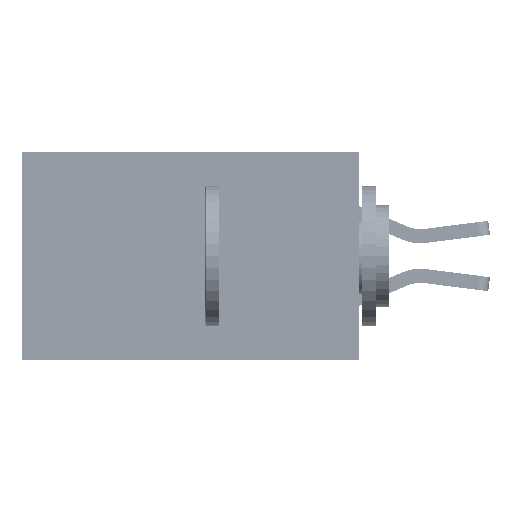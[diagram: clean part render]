
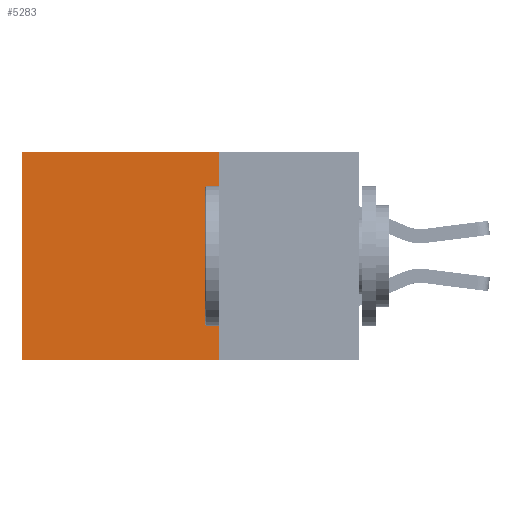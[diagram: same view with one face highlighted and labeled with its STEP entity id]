
A CAD part, left-side view. The second image highlights one B-rep face of the part: STEP entity #5283.
In plain terms, the highlighted planar face has unit normal (-1, 0, 0).
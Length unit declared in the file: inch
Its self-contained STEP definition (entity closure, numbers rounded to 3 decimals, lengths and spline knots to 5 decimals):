
#242 = VERTEX_POINT ( 'NONE', #3728 ) ;
#617 = FACE_OUTER_BOUND ( 'NONE', #26051, .T. ) ;
#1172 = EDGE_CURVE ( 'NONE', #27833, #26442, #19711, .T. ) ;
#1652 = VECTOR ( 'NONE', #17837, 39.37008 ) ;
#2261 = CARTESIAN_POINT ( 'NONE',  ( 0.2875, 0.25, -0.37 ) ) ;
#3349 = VECTOR ( 'NONE', #19250, 39.37008 ) ;
#3728 = CARTESIAN_POINT ( 'NONE',  ( 0.2875, 0.6, 0. ) ) ;
#4621 = DIRECTION ( 'NONE',  ( 0., 0., -1. ) ) ;
#5283 = ADVANCED_FACE ( 'NONE', ( #617 ), #14003, .F. ) ;
#5705 = DIRECTION ( 'NONE',  ( 1., 0., 0. ) ) ;
#5849 = EDGE_CURVE ( 'NONE', #26442, #14584, #29933, .T. ) ;
#10120 = VECTOR ( 'NONE', #17584, 39.37008 ) ;
#10176 = EDGE_CURVE ( 'NONE', #242, #14584, #37943, .T. ) ;
#12359 = DIRECTION ( 'NONE',  ( 0., 0., -1. ) ) ;
#14003 = PLANE ( 'NONE',  #40813 ) ;
#14584 = VERTEX_POINT ( 'NONE', #40375 ) ;
#17404 = ORIENTED_EDGE ( 'NONE', *, *, #31392, .T. ) ;
#17584 = DIRECTION ( 'NONE',  ( 0., 1., 0. ) ) ;
#17837 = DIRECTION ( 'NONE',  ( 0., 1., 0. ) ) ;
#18620 = LINE ( 'NONE', #33529, #10120 ) ;
#19250 = DIRECTION ( 'NONE',  ( 0., 0., -1. ) ) ;
#19290 = CARTESIAN_POINT ( 'NONE',  ( 0.2875, 0.25, -0.37 ) ) ;
#19711 = LINE ( 'NONE', #36490, #3349 ) ;
#23425 = ORIENTED_EDGE ( 'NONE', *, *, #1172, .F. ) ;
#26051 = EDGE_LOOP ( 'NONE', ( #35237, #38483, #23425, #17404 ) ) ;
#26442 = VERTEX_POINT ( 'NONE', #19290 ) ;
#26561 = CARTESIAN_POINT ( 'NONE',  ( 0.2875, 0.25, 0. ) ) ;
#27833 = VERTEX_POINT ( 'NONE', #26561 ) ;
#29933 = LINE ( 'NONE', #2261, #1652 ) ;
#31392 = EDGE_CURVE ( 'NONE', #27833, #242, #18620, .T. ) ;
#33529 = CARTESIAN_POINT ( 'NONE',  ( 0.2875, 0.25, 0. ) ) ;
#35237 = ORIENTED_EDGE ( 'NONE', *, *, #10176, .T. ) ;
#36490 = CARTESIAN_POINT ( 'NONE',  ( 0.2875, 0.25, 0. ) ) ;
#36962 = VECTOR ( 'NONE', #4621, 39.37008 ) ;
#37098 = CARTESIAN_POINT ( 'NONE',  ( 0.2875, 0.25, 0. ) ) ;
#37943 = LINE ( 'NONE', #39884, #36962 ) ;
#38483 = ORIENTED_EDGE ( 'NONE', *, *, #5849, .F. ) ;
#39884 = CARTESIAN_POINT ( 'NONE',  ( 0.2875, 0.6, 0. ) ) ;
#40375 = CARTESIAN_POINT ( 'NONE',  ( 0.2875, 0.6, -0.37 ) ) ;
#40813 = AXIS2_PLACEMENT_3D ( 'NONE', #37098, #5705, #12359 ) ;
